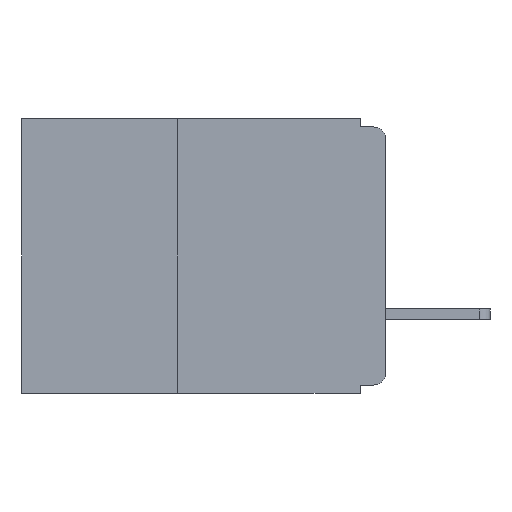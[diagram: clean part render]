
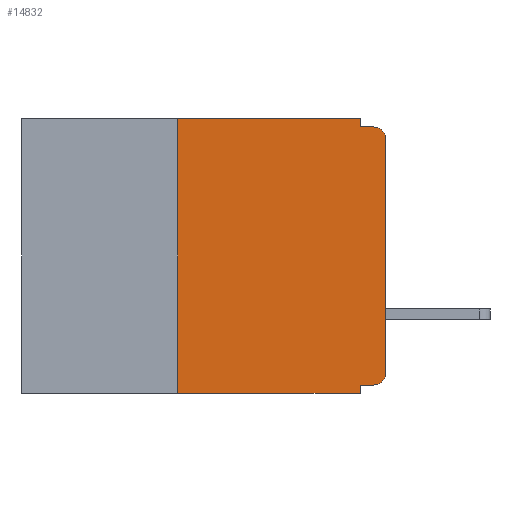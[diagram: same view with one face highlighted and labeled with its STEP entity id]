
A CAD part, left-side view. The second image highlights one B-rep face of the part: STEP entity #14832.
In plain terms, the highlighted planar face has unit normal (-1, 0, 0).
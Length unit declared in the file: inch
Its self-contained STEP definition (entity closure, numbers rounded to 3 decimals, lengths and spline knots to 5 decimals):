
#707 = ORIENTED_EDGE ( 'NONE', *, *, #25520, .F. ) ;
#2181 = CARTESIAN_POINT ( 'NONE',  ( 0., 0.25, -0.33 ) ) ;
#2415 = EDGE_CURVE ( 'NONE', #7674, #7705, #5685, .T. ) ;
#2555 = VERTEX_POINT ( 'NONE', #2847 ) ;
#2847 = CARTESIAN_POINT ( 'NONE',  ( 0., 0.015, -0.32 ) ) ;
#3273 = CARTESIAN_POINT ( 'NONE',  ( 0., 0.031, -0.32 ) ) ;
#3864 = AXIS2_PLACEMENT_3D ( 'NONE', #4235, #19680, #6472 ) ;
#4235 = CARTESIAN_POINT ( 'NONE',  ( 0., 0.015, -0.025 ) ) ;
#4275 = VECTOR ( 'NONE', #4901, 39.37008 ) ;
#4411 = LINE ( 'NONE', #10402, #21349 ) ;
#4793 = CIRCLE ( 'NONE', #3864, 0.015 ) ;
#4901 = DIRECTION ( 'NONE',  ( 0., 0., -1. ) ) ;
#5602 = ORIENTED_EDGE ( 'NONE', *, *, #18448, .F. ) ;
#5685 = LINE ( 'NONE', #25456, #28402 ) ;
#6373 = VERTEX_POINT ( 'NONE', #23708 ) ;
#6472 = DIRECTION ( 'NONE',  ( 0., 0., -1. ) ) ;
#6647 = ORIENTED_EDGE ( 'NONE', *, *, #15288, .T. ) ;
#6693 = VERTEX_POINT ( 'NONE', #26976 ) ;
#7674 = VERTEX_POINT ( 'NONE', #25855 ) ;
#7705 = VERTEX_POINT ( 'NONE', #23252 ) ;
#8598 = FACE_OUTER_BOUND ( 'NONE', #19648, .T. ) ;
#8602 = VECTOR ( 'NONE', #26359, 39.37008 ) ;
#9135 = CARTESIAN_POINT ( 'NONE',  ( 0., 0.015, -0.305 ) ) ;
#9318 = CARTESIAN_POINT ( 'NONE',  ( 0., 0.437, -0.33 ) ) ;
#9494 = VERTEX_POINT ( 'NONE', #18590 ) ;
#10402 = CARTESIAN_POINT ( 'NONE',  ( 0., 0., -0.32 ) ) ;
#11350 = DIRECTION ( 'NONE',  ( 1., 0., 0. ) ) ;
#11386 = DIRECTION ( 'NONE',  ( 0., 0., -1. ) ) ;
#11562 = DIRECTION ( 'NONE',  ( 0., -1., 0. ) ) ;
#11614 = AXIS2_PLACEMENT_3D ( 'NONE', #24507, #11350, #26703 ) ;
#11989 = VERTEX_POINT ( 'NONE', #21952 ) ;
#12632 = DIRECTION ( 'NONE',  ( 0., 1., 0. ) ) ;
#12854 = CARTESIAN_POINT ( 'NONE',  ( 0., 0.25, 0. ) ) ;
#13510 = ORIENTED_EDGE ( 'NONE', *, *, #2415, .F. ) ;
#13870 = LINE ( 'NONE', #17710, #24901 ) ;
#14081 = VECTOR ( 'NONE', #22085, 39.37008 ) ;
#14255 = EDGE_CURVE ( 'NONE', #2555, #6693, #25861, .T. ) ;
#14275 = VECTOR ( 'NONE', #11562, 39.37008 ) ;
#14458 = VERTEX_POINT ( 'NONE', #3273 ) ;
#14832 = ADVANCED_FACE ( 'NONE', ( #8598 ), #22272, .F. ) ;
#14947 = LINE ( 'NONE', #9318, #14275 ) ;
#15126 = LINE ( 'NONE', #21928, #8602 ) ;
#15288 = EDGE_CURVE ( 'NONE', #6693, #11989, #13870, .T. ) ;
#15785 = ORIENTED_EDGE ( 'NONE', *, *, #16837, .F. ) ;
#16265 = EDGE_CURVE ( 'NONE', #2555, #14458, #4411, .T. ) ;
#16837 = EDGE_CURVE ( 'NONE', #14458, #6373, #23078, .T. ) ;
#17710 = CARTESIAN_POINT ( 'NONE',  ( 0., 0., 0. ) ) ;
#17856 = VECTOR ( 'NONE', #21504, 39.37008 ) ;
#18138 = CARTESIAN_POINT ( 'NONE',  ( 0., 0.031, 0. ) ) ;
#18448 = EDGE_CURVE ( 'NONE', #24887, #7674, #21214, .T. ) ;
#18590 = CARTESIAN_POINT ( 'NONE',  ( 0., 0.25, -0.33 ) ) ;
#18891 = ORIENTED_EDGE ( 'NONE', *, *, #24882, .F. ) ;
#19648 = EDGE_LOOP ( 'NONE', ( #6647, #27822, #13510, #5602, #18891, #707, #25512, #15785, #26760, #20788 ) ) ;
#19680 = DIRECTION ( 'NONE',  ( -1., 0., 0. ) ) ;
#19712 = CARTESIAN_POINT ( 'NONE',  ( 0., 0.031, 0. ) ) ;
#19902 = LINE ( 'NONE', #2181, #14081 ) ;
#20788 = ORIENTED_EDGE ( 'NONE', *, *, #14255, .T. ) ;
#20839 = VERTEX_POINT ( 'NONE', #12854 ) ;
#21214 = LINE ( 'NONE', #18138, #4275 ) ;
#21349 = VECTOR ( 'NONE', #12632, 39.37008 ) ;
#21504 = DIRECTION ( 'NONE',  ( 0., 0., -1. ) ) ;
#21928 = CARTESIAN_POINT ( 'NONE',  ( 0., 0.437, 0. ) ) ;
#21952 = CARTESIAN_POINT ( 'NONE',  ( 0., 0., -0.025 ) ) ;
#22085 = DIRECTION ( 'NONE',  ( 0., 0., 1. ) ) ;
#22164 = DIRECTION ( 'NONE',  ( 0., 0., 1. ) ) ;
#22272 = PLANE ( 'NONE',  #11614 ) ;
#23078 = LINE ( 'NONE', #23650, #17856 ) ;
#23252 = CARTESIAN_POINT ( 'NONE',  ( 0., 0.015, -0.01 ) ) ;
#23650 = CARTESIAN_POINT ( 'NONE',  ( 0., 0.031, -0.33 ) ) ;
#23708 = CARTESIAN_POINT ( 'NONE',  ( 0., 0.031, -0.33 ) ) ;
#23937 = EDGE_CURVE ( 'NONE', #11989, #7705, #4793, .T. ) ;
#24507 = CARTESIAN_POINT ( 'NONE',  ( 0., 0.437, 0. ) ) ;
#24548 = DIRECTION ( 'NONE',  ( -1., 0., 0. ) ) ;
#24882 = EDGE_CURVE ( 'NONE', #20839, #24887, #15126, .T. ) ;
#24887 = VERTEX_POINT ( 'NONE', #19712 ) ;
#24901 = VECTOR ( 'NONE', #22164, 39.37008 ) ;
#25314 = DIRECTION ( 'NONE',  ( 0., -1., 0. ) ) ;
#25456 = CARTESIAN_POINT ( 'NONE',  ( 0., 0., -0.01 ) ) ;
#25512 = ORIENTED_EDGE ( 'NONE', *, *, #28061, .T. ) ;
#25520 = EDGE_CURVE ( 'NONE', #9494, #20839, #19902, .T. ) ;
#25855 = CARTESIAN_POINT ( 'NONE',  ( 0., 0.031, -0.01 ) ) ;
#25861 = CIRCLE ( 'NONE', #26498, 0.015 ) ;
#26359 = DIRECTION ( 'NONE',  ( 0., -1., 0. ) ) ;
#26498 = AXIS2_PLACEMENT_3D ( 'NONE', #9135, #24548, #11386 ) ;
#26703 = DIRECTION ( 'NONE',  ( 0., 0., -1. ) ) ;
#26760 = ORIENTED_EDGE ( 'NONE', *, *, #16265, .F. ) ;
#26976 = CARTESIAN_POINT ( 'NONE',  ( 0., 0., -0.305 ) ) ;
#27822 = ORIENTED_EDGE ( 'NONE', *, *, #23937, .T. ) ;
#28061 = EDGE_CURVE ( 'NONE', #9494, #6373, #14947, .T. ) ;
#28402 = VECTOR ( 'NONE', #25314, 39.37008 ) ;
